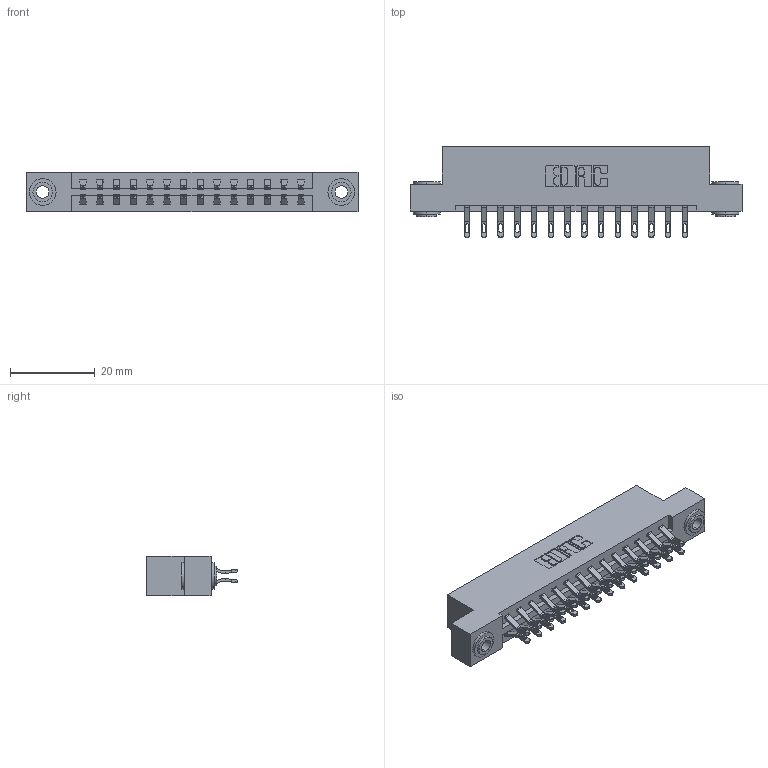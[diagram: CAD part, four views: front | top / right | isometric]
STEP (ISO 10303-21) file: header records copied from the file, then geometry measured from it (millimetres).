
FILE_DESCRIPTION (( 'STEP AP203' ), '1' );
FILE_NAME ('337-028-555-203.STEP', '2019-10-08T17:13:42', ( '' ), ( '' ), 'SwSTEP 2.0', 'SolidWorks 2016', '' );
FILE_SCHEMA (( 'CONFIG_CONTROL_DESIGN' ));
Length unit declared in the file: inch
Products named in the file (4): 337-028-555-203; 337 Part_Flush Mounting Lugs - 0.156 Dia-TH; 345-292-001_555 Tail; 345-250-002_345-250-002-102
Assembly tree (31 placements, depth 2):
  337-028-555-203
    337 Part_Flush Mounting Lugs - 0.156 Dia-TH
    345-292-001_555 Tail  x28
    345-250-002_345-250-002-102  x2
Bounding box: 78.49 x 21.47 x 9.4 mm (x, y, z)
Volume: 7999.4 mm3; surface area: 9301.8 mm2
Topology: 31 solids, 31 shells, 1832 faces, 5679 edges, 3782 vertices
Faces by surface type: plane 1088, cylinder 736, cone 8
Entity records: 15452 total; most frequent: CARTESIAN_POINT 2635, ORIENTED_EDGE 2534, DIRECTION 2297, EDGE_CURVE 1267, LINE 1095, VECTOR 1095, VERTEX_POINT 842, AXIS2_PLACEMENT_3D 601
